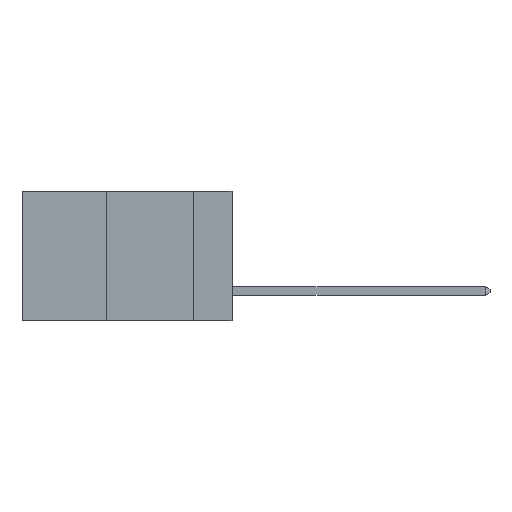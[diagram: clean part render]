
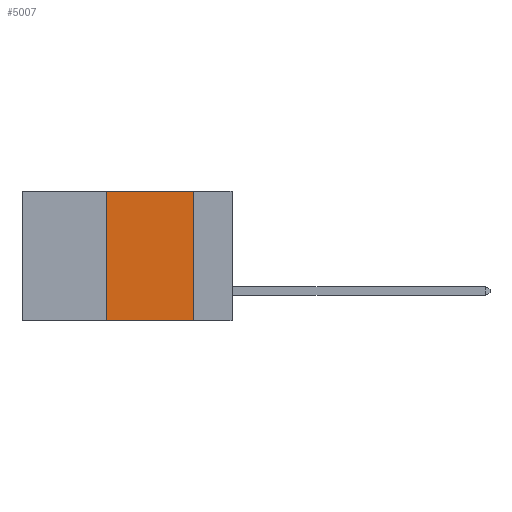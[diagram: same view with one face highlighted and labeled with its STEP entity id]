
A CAD part, left-side view. The second image highlights one B-rep face of the part: STEP entity #5007.
In plain terms, the highlighted planar face has unit normal (-1, 0, 0).
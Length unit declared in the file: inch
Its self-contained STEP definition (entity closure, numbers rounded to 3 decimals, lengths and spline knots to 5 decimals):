
#2654 = CARTESIAN_POINT ( 'NONE',  ( 0., 0.11, -0.37 ) ) ;
#3598 = DIRECTION ( 'NONE',  ( 1., 0., 0. ) ) ;
#3941 = AXIS2_PLACEMENT_3D ( 'NONE', #14051, #3598, #15748 ) ;
#3997 = LINE ( 'NONE', #12813, #21686 ) ;
#4232 = ORIENTED_EDGE ( 'NONE', *, *, #12767, .F. ) ;
#4327 = EDGE_LOOP ( 'NONE', ( #19599, #10630, #4232, #8500 ) ) ;
#4912 = EDGE_CURVE ( 'NONE', #19704, #15879, #12848, .T. ) ;
#5007 = ADVANCED_FACE ( 'NONE', ( #11816 ), #10679, .F. ) ;
#5964 = DIRECTION ( 'NONE',  ( 0., 0., 1. ) ) ;
#7261 = EDGE_CURVE ( 'NONE', #20863, #19704, #20030, .T. ) ;
#8500 = ORIENTED_EDGE ( 'NONE', *, *, #20343, .T. ) ;
#9380 = CARTESIAN_POINT ( 'NONE',  ( 0., 0.36, 0. ) ) ;
#9456 = CARTESIAN_POINT ( 'NONE',  ( 0., 0.36, -0.37 ) ) ;
#10203 = LINE ( 'NONE', #19715, #14156 ) ;
#10630 = ORIENTED_EDGE ( 'NONE', *, *, #7261, .F. ) ;
#10679 = PLANE ( 'NONE',  #3941 ) ;
#11042 = VERTEX_POINT ( 'NONE', #9456 ) ;
#11241 = DIRECTION ( 'NONE',  ( 0., -1., 0. ) ) ;
#11816 = FACE_OUTER_BOUND ( 'NONE', #4327, .T. ) ;
#12324 = VECTOR ( 'NONE', #15528, 39.37008 ) ;
#12767 = EDGE_CURVE ( 'NONE', #11042, #20863, #3997, .T. ) ;
#12813 = CARTESIAN_POINT ( 'NONE',  ( 0., 0.36, 0. ) ) ;
#12848 = LINE ( 'NONE', #13822, #12324 ) ;
#13287 = DIRECTION ( 'NONE',  ( 0., -1., 0. ) ) ;
#13822 = CARTESIAN_POINT ( 'NONE',  ( 0., 0.11, 0. ) ) ;
#14051 = CARTESIAN_POINT ( 'NONE',  ( 0., 0.6, 0. ) ) ;
#14156 = VECTOR ( 'NONE', #11241, 39.37008 ) ;
#15528 = DIRECTION ( 'NONE',  ( 0., 0., -1. ) ) ;
#15543 = VECTOR ( 'NONE', #13287, 39.37008 ) ;
#15748 = DIRECTION ( 'NONE',  ( 0., 0., -1. ) ) ;
#15879 = VERTEX_POINT ( 'NONE', #2654 ) ;
#18304 = CARTESIAN_POINT ( 'NONE',  ( 0., 0.6, 0. ) ) ;
#19599 = ORIENTED_EDGE ( 'NONE', *, *, #4912, .F. ) ;
#19704 = VERTEX_POINT ( 'NONE', #21034 ) ;
#19715 = CARTESIAN_POINT ( 'NONE',  ( 0., 0.6, -0.37 ) ) ;
#20030 = LINE ( 'NONE', #18304, #15543 ) ;
#20343 = EDGE_CURVE ( 'NONE', #11042, #15879, #10203, .T. ) ;
#20863 = VERTEX_POINT ( 'NONE', #9380 ) ;
#21034 = CARTESIAN_POINT ( 'NONE',  ( 0., 0.11, 0. ) ) ;
#21686 = VECTOR ( 'NONE', #5964, 39.37008 ) ;
